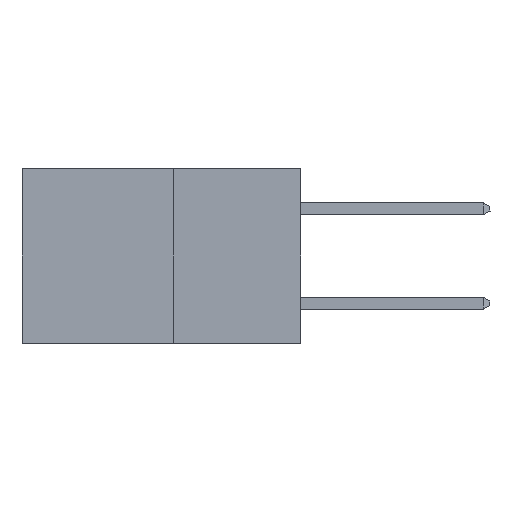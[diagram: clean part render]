
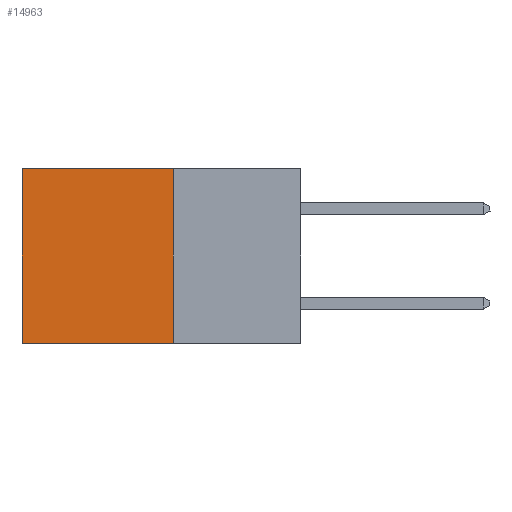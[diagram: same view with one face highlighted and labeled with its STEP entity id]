
A CAD part, left-side view. The second image highlights one B-rep face of the part: STEP entity #14963.
In plain terms, the highlighted planar face has unit normal (-1, 0, 0).
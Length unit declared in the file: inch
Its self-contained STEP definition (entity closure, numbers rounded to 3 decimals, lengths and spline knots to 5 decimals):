
#1642 = EDGE_CURVE ( 'NONE', #14162, #13297, #3280, .T. ) ;
#1761 = DIRECTION ( 'NONE',  ( 0., 1., 0. ) ) ;
#1908 = CARTESIAN_POINT ( 'NONE',  ( 0.277, 0.59, 0. ) ) ;
#1932 = CARTESIAN_POINT ( 'NONE',  ( 0.277, 0.27, 0. ) ) ;
#2202 = EDGE_CURVE ( 'NONE', #7377, #7008, #7531, .T. ) ;
#2856 = VECTOR ( 'NONE', #11418, 39.37008 ) ;
#3094 = VECTOR ( 'NONE', #10330, 39.37008 ) ;
#3280 = LINE ( 'NONE', #8257, #2856 ) ;
#3305 = CARTESIAN_POINT ( 'NONE',  ( 0.277, 0.27, -0.37 ) ) ;
#6143 = VECTOR ( 'NONE', #10176, 39.37008 ) ;
#6310 = DIRECTION ( 'NONE',  ( 0., 0., -1. ) ) ;
#7008 = VERTEX_POINT ( 'NONE', #1908 ) ;
#7021 = ORIENTED_EDGE ( 'NONE', *, *, #11010, .F. ) ;
#7377 = VERTEX_POINT ( 'NONE', #8107 ) ;
#7436 = ORIENTED_EDGE ( 'NONE', *, *, #8348, .T. ) ;
#7531 = LINE ( 'NONE', #1932, #14837 ) ;
#8107 = CARTESIAN_POINT ( 'NONE',  ( 0.277, 0.27, 0. ) ) ;
#8257 = CARTESIAN_POINT ( 'NONE',  ( 0.277, 0.27, -0.37 ) ) ;
#8348 = EDGE_CURVE ( 'NONE', #7008, #13297, #17621, .T. ) ;
#8365 = CARTESIAN_POINT ( 'NONE',  ( 0.277, 0.59, -0.37 ) ) ;
#8792 = CARTESIAN_POINT ( 'NONE',  ( 0.277, 0.27, -0.37 ) ) ;
#9663 = EDGE_LOOP ( 'NONE', ( #7436, #15834, #7021, #10714 ) ) ;
#10176 = DIRECTION ( 'NONE',  ( 0., 0., -1. ) ) ;
#10330 = DIRECTION ( 'NONE',  ( 0., 0., -1. ) ) ;
#10714 = ORIENTED_EDGE ( 'NONE', *, *, #2202, .T. ) ;
#11010 = EDGE_CURVE ( 'NONE', #7377, #14162, #17039, .T. ) ;
#11418 = DIRECTION ( 'NONE',  ( 0., 1., 0. ) ) ;
#11816 = PLANE ( 'NONE',  #16144 ) ;
#12069 = FACE_OUTER_BOUND ( 'NONE', #9663, .T. ) ;
#13191 = CARTESIAN_POINT ( 'NONE',  ( 0.277, 0.27, -0.37 ) ) ;
#13297 = VERTEX_POINT ( 'NONE', #8365 ) ;
#14162 = VERTEX_POINT ( 'NONE', #3305 ) ;
#14516 = DIRECTION ( 'NONE',  ( 1., 0., 0. ) ) ;
#14837 = VECTOR ( 'NONE', #1761, 39.37008 ) ;
#14963 = ADVANCED_FACE ( 'NONE', ( #12069 ), #11816, .F. ) ;
#15834 = ORIENTED_EDGE ( 'NONE', *, *, #1642, .F. ) ;
#16144 = AXIS2_PLACEMENT_3D ( 'NONE', #13191, #14516, #6310 ) ;
#17039 = LINE ( 'NONE', #8792, #6143 ) ;
#17099 = CARTESIAN_POINT ( 'NONE',  ( 0.277, 0.59, -0.37 ) ) ;
#17621 = LINE ( 'NONE', #17099, #3094 ) ;
